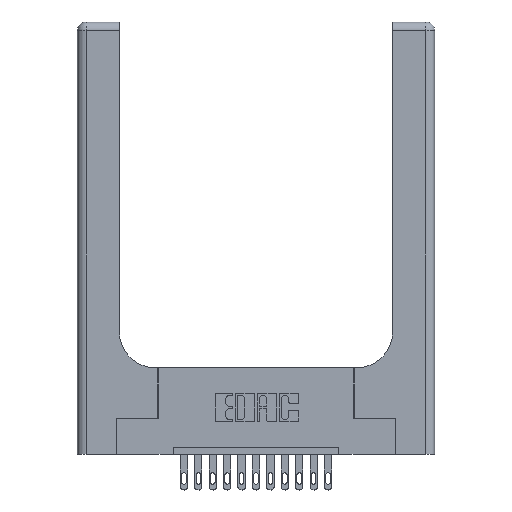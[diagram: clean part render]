
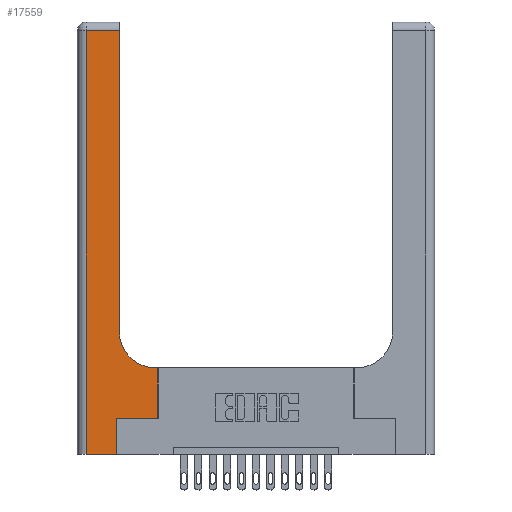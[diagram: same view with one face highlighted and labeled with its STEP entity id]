
A CAD part, top view. The second image highlights one B-rep face of the part: STEP entity #17559.
In plain terms, the highlighted planar face has unit normal (0, 0, 1).
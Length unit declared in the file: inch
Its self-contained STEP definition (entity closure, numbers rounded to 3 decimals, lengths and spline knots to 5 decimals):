
#477 = CARTESIAN_POINT ( 'NONE',  ( 0., 3., 0.37 ) ) ;
#612 = CARTESIAN_POINT ( 'NONE',  ( 0.269, 0., 0.37 ) ) ;
#1018 = VECTOR ( 'NONE', #3194, 39.37008 ) ;
#1029 = ORIENTED_EDGE ( 'NONE', *, *, #16586, .T. ) ;
#1232 = VERTEX_POINT ( 'NONE', #4613 ) ;
#1535 = EDGE_CURVE ( 'NONE', #8385, #12049, #9813, .T. ) ;
#1611 = PLANE ( 'NONE',  #13136 ) ;
#2309 = LINE ( 'NONE', #16690, #1018 ) ;
#2426 = EDGE_CURVE ( 'NONE', #1232, #5810, #7674, .T. ) ;
#2651 = CARTESIAN_POINT ( 'NONE',  ( 0.5415, 0.85, 0.37 ) ) ;
#2789 = VECTOR ( 'NONE', #4446, 39.37008 ) ;
#3194 = DIRECTION ( 'NONE',  ( -1., 0., 0. ) ) ;
#3373 = VERTEX_POINT ( 'NONE', #7978 ) ;
#3713 = VERTEX_POINT ( 'NONE', #12305 ) ;
#4193 = VERTEX_POINT ( 'NONE', #6406 ) ;
#4381 = VECTOR ( 'NONE', #9193, 39.37008 ) ;
#4446 = DIRECTION ( 'NONE',  ( 1., 0., 0. ) ) ;
#4537 = DIRECTION ( 'NONE',  ( -1., 0., 0. ) ) ;
#4613 = CARTESIAN_POINT ( 'NONE',  ( 0.06, 0., 0.37 ) ) ;
#4991 = EDGE_CURVE ( 'NONE', #12049, #4193, #11001, .T. ) ;
#5102 = VECTOR ( 'NONE', #14372, 39.37008 ) ;
#5312 = CARTESIAN_POINT ( 'NONE',  ( 0.2915, 2.94, 0.37 ) ) ;
#5525 = CIRCLE ( 'NONE', #7711, 0.25 ) ;
#5810 = VERTEX_POINT ( 'NONE', #612 ) ;
#5954 = CARTESIAN_POINT ( 'NONE',  ( 0.269, 0., 0.37 ) ) ;
#6218 = VECTOR ( 'NONE', #14788, 39.37008 ) ;
#6406 = CARTESIAN_POINT ( 'NONE',  ( 0.5585, 0.6, 0.37 ) ) ;
#6793 = EDGE_LOOP ( 'NONE', ( #9081, #10764, #15645, #7331, #1029, #8821, #14272, #7429, #8676 ) ) ;
#7222 = DIRECTION ( 'NONE',  ( 0., 1., 0. ) ) ;
#7331 = ORIENTED_EDGE ( 'NONE', *, *, #2426, .T. ) ;
#7429 = ORIENTED_EDGE ( 'NONE', *, *, #8538, .T. ) ;
#7674 = LINE ( 'NONE', #13809, #2789 ) ;
#7681 = CARTESIAN_POINT ( 'NONE',  ( 0.5585, 0.25, 0.37 ) ) ;
#7711 = AXIS2_PLACEMENT_3D ( 'NONE', #2651, #9535, #9353 ) ;
#7928 = CARTESIAN_POINT ( 'NONE',  ( 0.2915, 0.6, 0.37 ) ) ;
#7978 = CARTESIAN_POINT ( 'NONE',  ( 0.2915, 0.85, 0.37 ) ) ;
#7987 = DIRECTION ( 'NONE',  ( -1., 0., 0. ) ) ;
#8256 = VERTEX_POINT ( 'NONE', #5312 ) ;
#8385 = VERTEX_POINT ( 'NONE', #13935 ) ;
#8538 = EDGE_CURVE ( 'NONE', #4193, #3713, #10251, .T. ) ;
#8676 = ORIENTED_EDGE ( 'NONE', *, *, #16258, .T. ) ;
#8777 = CARTESIAN_POINT ( 'NONE',  ( 0.06, 3., 0.37 ) ) ;
#8821 = ORIENTED_EDGE ( 'NONE', *, *, #1535, .T. ) ;
#9081 = ORIENTED_EDGE ( 'NONE', *, *, #17025, .T. ) ;
#9193 = DIRECTION ( 'NONE',  ( 0., -1., 0. ) ) ;
#9353 = DIRECTION ( 'NONE',  ( 1., 0., 0. ) ) ;
#9535 = DIRECTION ( 'NONE',  ( 0., 0., -1. ) ) ;
#9813 = LINE ( 'NONE', #17410, #6218 ) ;
#9971 = DIRECTION ( 'NONE',  ( 0., 0., -1. ) ) ;
#10150 = CARTESIAN_POINT ( 'NONE',  ( 0.5585, 0.25, 0.37 ) ) ;
#10251 = LINE ( 'NONE', #7928, #10677 ) ;
#10313 = LINE ( 'NONE', #5954, #16888 ) ;
#10577 = EDGE_CURVE ( 'NONE', #14052, #1232, #14298, .T. ) ;
#10677 = VECTOR ( 'NONE', #7987, 39.37008 ) ;
#10716 = LINE ( 'NONE', #14222, #15386 ) ;
#10764 = ORIENTED_EDGE ( 'NONE', *, *, #15887, .T. ) ;
#11001 = LINE ( 'NONE', #10150, #5102 ) ;
#12049 = VERTEX_POINT ( 'NONE', #7681 ) ;
#12305 = CARTESIAN_POINT ( 'NONE',  ( 0.5415, 0.6, 0.37 ) ) ;
#12876 = DIRECTION ( 'NONE',  ( 0., 1., 0. ) ) ;
#13136 = AXIS2_PLACEMENT_3D ( 'NONE', #477, #9971, #4537 ) ;
#13809 = CARTESIAN_POINT ( 'NONE',  ( 0., 0., 0.37 ) ) ;
#13935 = CARTESIAN_POINT ( 'NONE',  ( 0.269, 0.25, 0.37 ) ) ;
#14052 = VERTEX_POINT ( 'NONE', #14267 ) ;
#14222 = CARTESIAN_POINT ( 'NONE',  ( 0.2915, 3., 0.37 ) ) ;
#14267 = CARTESIAN_POINT ( 'NONE',  ( 0.06, 2.94, 0.37 ) ) ;
#14272 = ORIENTED_EDGE ( 'NONE', *, *, #4991, .T. ) ;
#14298 = LINE ( 'NONE', #8777, #4381 ) ;
#14372 = DIRECTION ( 'NONE',  ( 0., 1., 0. ) ) ;
#14788 = DIRECTION ( 'NONE',  ( 1., 0., 0. ) ) ;
#15353 = FACE_OUTER_BOUND ( 'NONE', #6793, .T. ) ;
#15386 = VECTOR ( 'NONE', #12876, 39.37008 ) ;
#15645 = ORIENTED_EDGE ( 'NONE', *, *, #10577, .T. ) ;
#15887 = EDGE_CURVE ( 'NONE', #8256, #14052, #2309, .T. ) ;
#16258 = EDGE_CURVE ( 'NONE', #3713, #3373, #5525, .T. ) ;
#16586 = EDGE_CURVE ( 'NONE', #5810, #8385, #10313, .T. ) ;
#16690 = CARTESIAN_POINT ( 'NONE',  ( 0., 2.94, 0.37 ) ) ;
#16888 = VECTOR ( 'NONE', #7222, 39.37008 ) ;
#17025 = EDGE_CURVE ( 'NONE', #3373, #8256, #10716, .T. ) ;
#17410 = CARTESIAN_POINT ( 'NONE',  ( 0.269, 0.25, 0.37 ) ) ;
#17559 = ADVANCED_FACE ( 'NONE', ( #15353 ), #1611, .F. ) ;
